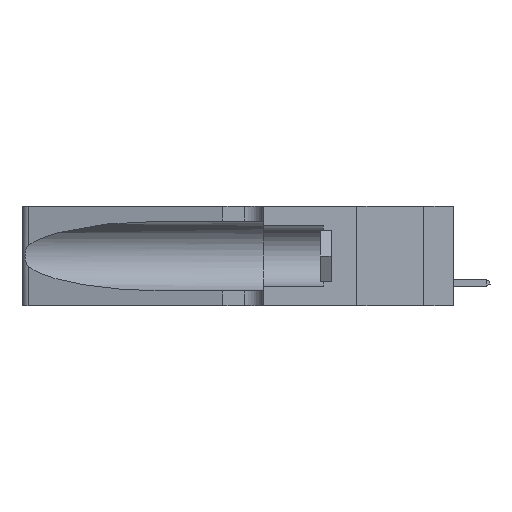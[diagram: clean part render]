
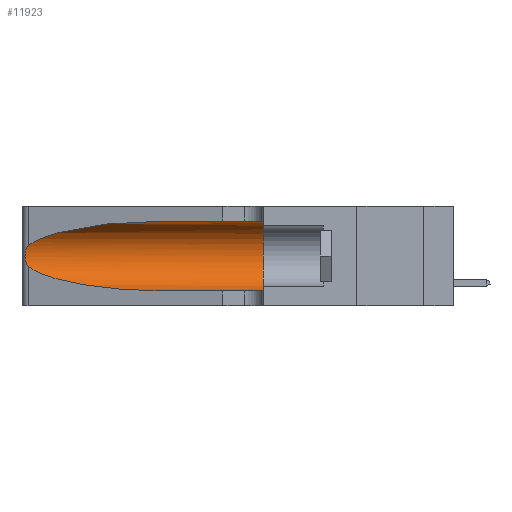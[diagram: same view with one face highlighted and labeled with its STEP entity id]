
A CAD part, left-side view. The second image highlights one B-rep face of the part: STEP entity #11923.
In plain terms, the highlighted cylindrical face has radius 3.308 mm (diameter 6.617 mm), a partial arc.
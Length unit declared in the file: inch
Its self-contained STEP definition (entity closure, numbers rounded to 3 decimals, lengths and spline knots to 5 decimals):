
#894 = VERTEX_POINT ( 'NONE', #18241 ) ;
#2662 = ORIENTED_EDGE ( 'NONE', *, *, #11998, .T. ) ;
#3716 = CARTESIAN_POINT ( 'NONE',  ( 0.1305, 1.61858, 0.31525 ) ) ;
#3843 = CARTESIAN_POINT ( 'NONE',  ( 0.25639, 1.23184, 0.21858 ) ) ;
#4174 = VECTOR ( 'NONE', #13756, 39.37008 ) ;
#4624 = VERTEX_POINT ( 'NONE', #19891 ) ;
#5627 =( BOUNDED_CURVE ( )  B_SPLINE_CURVE ( 3, ( #22810, #22242, #10657, #18251 ),
 .UNSPECIFIED., .F., .T. ) 
 B_SPLINE_CURVE_WITH_KNOTS ( ( 4, 4 ),
 ( 3.44316, 4.71239 ),
 .UNSPECIFIED. ) 
 CURVE ( )  GEOMETRIC_REPRESENTATION_ITEM ( )  RATIONAL_B_SPLINE_CURVE ( ( 1., 0.87, 0.87, 1. ) ) 
 REPRESENTATION_ITEM ( '' )  );
#6745 = VERTEX_POINT ( 'NONE', #7032 ) ;
#6784 = CARTESIAN_POINT ( 'NONE',  ( 0.26075, 1.23896, 0.19203 ) ) ;
#7032 = CARTESIAN_POINT ( 'NONE',  ( 0.25487, 1.22718, 0.14631 ) ) ;
#7461 = CYLINDRICAL_SURFACE ( 'NONE', #11515, 0.13025 ) ;
#7823 = ORIENTED_EDGE ( 'NONE', *, *, #21955, .T. ) ;
#8344 = LINE ( 'NONE', #23284, #31602 ) ;
#9040 = ORIENTED_EDGE ( 'NONE', *, *, #16693, .T. ) ;
#9173 = CARTESIAN_POINT ( 'NONE',  ( 0.25555, 1.22993, 0.14849 ) ) ;
#9221 = B_SPLINE_CURVE_WITH_KNOTS ( 'NONE', 3,
 ( #29670, #17154, #3843, #19513, #14578, #32391, #6784, #32146, #16814, #29789, #22324, #21869, #9173, #12021 ),
 .UNSPECIFIED., .F., .F.,
 ( 4, 2, 2, 2, 2, 2, 4 ),
 ( 0., 0.00027, 0.00053, 0.00107, 0.0016, 0.00187, 0.00214 ),
 .UNSPECIFIED. ) ;
#9962 = CARTESIAN_POINT ( 'NONE',  ( 0.18966, 0.96281, 0.31525 ) ) ;
#10334 = CARTESIAN_POINT ( 'NONE',  ( 0.1305, 0.35, 0.31525 ) ) ;
#10571 = VERTEX_POINT ( 'NONE', #16372 ) ;
#10657 = CARTESIAN_POINT ( 'NONE',  ( 0.18966, 0.96281, 0.05475 ) ) ;
#11515 = AXIS2_PLACEMENT_3D ( 'NONE', #29608, #16861, #19435 ) ;
#11843 = LINE ( 'NONE', #3716, #4174 ) ;
#11923 = ADVANCED_FACE ( 'NONE', ( #28710 ), #7461, .F. ) ;
#11998 = EDGE_CURVE ( 'NONE', #6745, #10571, #5627, .T. ) ;
#12021 = CARTESIAN_POINT ( 'NONE',  ( 0.25487, 1.22718, 0.14631 ) ) ;
#12396 = ORIENTED_EDGE ( 'NONE', *, *, #32078, .F. ) ;
#12547 = CARTESIAN_POINT ( 'NONE',  ( 0.2373, 1.15595, 0.28018 ) ) ;
#13337 = EDGE_LOOP ( 'NONE', ( #31264, #7823, #2662, #9040, #20401, #12396 ) ) ;
#13756 = DIRECTION ( 'NONE',  ( 0., -1., 0. ) ) ;
#14578 = CARTESIAN_POINT ( 'NONE',  ( 0.25854, 1.2359, 0.20912 ) ) ;
#16372 = CARTESIAN_POINT ( 'NONE',  ( 0.1305, 0.72297, 0.05475 ) ) ;
#16556 = DIRECTION ( 'NONE',  ( 0., 1., 0. ) ) ;
#16693 = EDGE_CURVE ( 'NONE', #10571, #18632, #8344, .T. ) ;
#16814 = CARTESIAN_POINT ( 'NONE',  ( 0.26017, 1.23833, 0.17102 ) ) ;
#16861 = DIRECTION ( 'NONE',  ( 0., -1., 0. ) ) ;
#17154 = CARTESIAN_POINT ( 'NONE',  ( 0.25555, 1.22994, 0.2215 ) ) ;
#17230 = EDGE_CURVE ( 'NONE', #894, #4624, #26028, .T. ) ;
#17851 = CARTESIAN_POINT ( 'NONE',  ( 0.1305, 0.35, 0.05475 ) ) ;
#18241 = CARTESIAN_POINT ( 'NONE',  ( 0.1305, 0.72297, 0.31525 ) ) ;
#18251 = CARTESIAN_POINT ( 'NONE',  ( 0.1305, 0.72297, 0.05475 ) ) ;
#18632 = VERTEX_POINT ( 'NONE', #17851 ) ;
#18756 = VERTEX_POINT ( 'NONE', #10334 ) ;
#19245 = DIRECTION ( 'NONE',  ( 0., 0., 1. ) ) ;
#19435 = DIRECTION ( 'NONE',  ( 0., 0., -1. ) ) ;
#19513 = CARTESIAN_POINT ( 'NONE',  ( 0.25787, 1.23484, 0.2124 ) ) ;
#19891 = CARTESIAN_POINT ( 'NONE',  ( 0.25487, 1.22718, 0.22369 ) ) ;
#20401 = ORIENTED_EDGE ( 'NONE', *, *, #29050, .F. ) ;
#20911 = DIRECTION ( 'NONE',  ( 0., -1., 0. ) ) ;
#21869 = CARTESIAN_POINT ( 'NONE',  ( 0.25639, 1.23186, 0.15144 ) ) ;
#21955 = EDGE_CURVE ( 'NONE', #4624, #6745, #9221, .T. ) ;
#22242 = CARTESIAN_POINT ( 'NONE',  ( 0.2373, 1.15595, 0.08982 ) ) ;
#22324 = CARTESIAN_POINT ( 'NONE',  ( 0.25789, 1.23486, 0.15765 ) ) ;
#22810 = CARTESIAN_POINT ( 'NONE',  ( 0.25487, 1.22718, 0.14631 ) ) ;
#23284 = CARTESIAN_POINT ( 'NONE',  ( 0.1305, 1.61858, 0.05475 ) ) ;
#24497 = CARTESIAN_POINT ( 'NONE',  ( 0.1305, 0.35, 0.185 ) ) ;
#24603 = CIRCLE ( 'NONE', #33151, 0.13025 ) ;
#25309 = CARTESIAN_POINT ( 'NONE',  ( 0.1305, 0.72297, 0.31525 ) ) ;
#26028 =( BOUNDED_CURVE ( )  B_SPLINE_CURVE ( 3, ( #25309, #9962, #12547, #30441 ),
 .UNSPECIFIED., .F., .F. ) 
 B_SPLINE_CURVE_WITH_KNOTS ( ( 4, 4 ),
 ( 1.5708, 2.84003 ),
 .UNSPECIFIED. ) 
 CURVE ( )  GEOMETRIC_REPRESENTATION_ITEM ( )  RATIONAL_B_SPLINE_CURVE ( ( 1., 0.87, 0.87, 1. ) ) 
 REPRESENTATION_ITEM ( '' )  );
#28710 = FACE_OUTER_BOUND ( 'NONE', #13337, .T. ) ;
#29050 = EDGE_CURVE ( 'NONE', #18756, #18632, #24603, .T. ) ;
#29608 = CARTESIAN_POINT ( 'NONE',  ( 0.1305, 1.61858, 0.185 ) ) ;
#29670 = CARTESIAN_POINT ( 'NONE',  ( 0.25487, 1.22718, 0.22369 ) ) ;
#29789 = CARTESIAN_POINT ( 'NONE',  ( 0.25856, 1.23593, 0.16098 ) ) ;
#30441 = CARTESIAN_POINT ( 'NONE',  ( 0.25487, 1.22718, 0.22369 ) ) ;
#31264 = ORIENTED_EDGE ( 'NONE', *, *, #17230, .T. ) ;
#31602 = VECTOR ( 'NONE', #20911, 39.37008 ) ;
#32078 = EDGE_CURVE ( 'NONE', #894, #18756, #11843, .T. ) ;
#32146 = CARTESIAN_POINT ( 'NONE',  ( 0.26075, 1.23896, 0.178 ) ) ;
#32391 = CARTESIAN_POINT ( 'NONE',  ( 0.26018, 1.23835, 0.19895 ) ) ;
#33151 = AXIS2_PLACEMENT_3D ( 'NONE', #24497, #16556, #19245 ) ;
